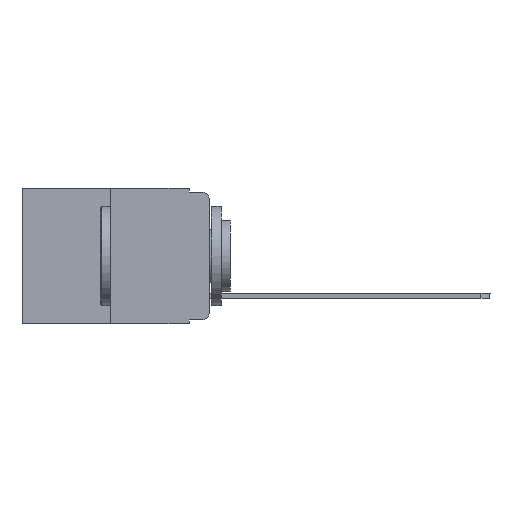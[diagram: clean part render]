
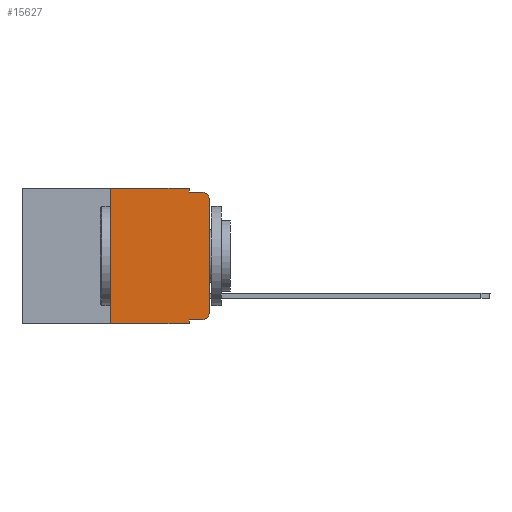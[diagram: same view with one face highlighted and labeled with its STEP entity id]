
A CAD part, left-side view. The second image highlights one B-rep face of the part: STEP entity #15627.
In plain terms, the highlighted planar face has unit normal (-1, 0, 0).
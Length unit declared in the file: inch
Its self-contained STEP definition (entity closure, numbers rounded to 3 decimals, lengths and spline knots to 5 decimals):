
#507 = CARTESIAN_POINT ( 'NONE',  ( 0., 0.051, 0. ) ) ;
#781 = EDGE_CURVE ( 'NONE', #1619, #7245, #6989, .T. ) ;
#1125 = DIRECTION ( 'NONE',  ( 0., 0., 1. ) ) ;
#1319 = VERTEX_POINT ( 'NONE', #2428 ) ;
#1418 = VECTOR ( 'NONE', #8610, 39.37008 ) ;
#1614 = ORIENTED_EDGE ( 'NONE', *, *, #6108, .T. ) ;
#1619 = VERTEX_POINT ( 'NONE', #7873 ) ;
#1660 = VERTEX_POINT ( 'NONE', #12229 ) ;
#1692 = VERTEX_POINT ( 'NONE', #3944 ) ;
#1760 = VECTOR ( 'NONE', #5339, 39.37008 ) ;
#1814 = EDGE_LOOP ( 'NONE', ( #13357, #5194, #2889, #8014, #16266, #16186, #7702, #11370, #1614, #3317 ) ) ;
#1961 = EDGE_CURVE ( 'NONE', #1660, #7245, #17568, .T. ) ;
#2119 = LINE ( 'NONE', #9915, #14086 ) ;
#2248 = EDGE_CURVE ( 'NONE', #11110, #13710, #10597, .T. ) ;
#2272 = CARTESIAN_POINT ( 'NONE',  ( 0., 0.473, -0.343 ) ) ;
#2428 = CARTESIAN_POINT ( 'NONE',  ( 0., 0.25, 0. ) ) ;
#2456 = FACE_OUTER_BOUND ( 'NONE', #1814, .T. ) ;
#2745 = CARTESIAN_POINT ( 'NONE',  ( 0., 0., -0.03 ) ) ;
#2828 = CARTESIAN_POINT ( 'NONE',  ( 0., 0.02, -0.01 ) ) ;
#2889 = ORIENTED_EDGE ( 'NONE', *, *, #11611, .F. ) ;
#3049 = VECTOR ( 'NONE', #4630, 39.37008 ) ;
#3073 = LINE ( 'NONE', #17088, #6129 ) ;
#3238 = LINE ( 'NONE', #5280, #1760 ) ;
#3317 = ORIENTED_EDGE ( 'NONE', *, *, #2248, .T. ) ;
#3724 = PLANE ( 'NONE',  #8675 ) ;
#3820 = AXIS2_PLACEMENT_3D ( 'NONE', #6805, #5267, #3923 ) ;
#3923 = DIRECTION ( 'NONE',  ( 0., 0., -1. ) ) ;
#3944 = CARTESIAN_POINT ( 'NONE',  ( 0., 0.051, -0.01 ) ) ;
#3973 = DIRECTION ( 'NONE',  ( 1., 0., 0. ) ) ;
#4630 = DIRECTION ( 'NONE',  ( 0., 0., -1. ) ) ;
#4683 = DIRECTION ( 'NONE',  ( 0., 0., -1. ) ) ;
#5143 = EDGE_CURVE ( 'NONE', #1319, #16774, #6836, .T. ) ;
#5194 = ORIENTED_EDGE ( 'NONE', *, *, #5973, .T. ) ;
#5267 = DIRECTION ( 'NONE',  ( -1., 0., 0. ) ) ;
#5280 = CARTESIAN_POINT ( 'NONE',  ( 0., 0.051, -0.01 ) ) ;
#5283 = VERTEX_POINT ( 'NONE', #2828 ) ;
#5339 = DIRECTION ( 'NONE',  ( 0., -1., 0. ) ) ;
#5973 = EDGE_CURVE ( 'NONE', #14614, #5283, #11148, .T. ) ;
#6108 = EDGE_CURVE ( 'NONE', #1619, #11110, #13962, .T. ) ;
#6129 = VECTOR ( 'NONE', #4683, 39.37008 ) ;
#6805 = CARTESIAN_POINT ( 'NONE',  ( 0., 0.02, -0.313 ) ) ;
#6836 = LINE ( 'NONE', #11260, #1418 ) ;
#6989 = LINE ( 'NONE', #507, #3049 ) ;
#7245 = VERTEX_POINT ( 'NONE', #16845 ) ;
#7702 = ORIENTED_EDGE ( 'NONE', *, *, #1961, .T. ) ;
#7873 = CARTESIAN_POINT ( 'NONE',  ( 0., 0.051, -0.333 ) ) ;
#7917 = DIRECTION ( 'NONE',  ( 0., -1., 0. ) ) ;
#8014 = ORIENTED_EDGE ( 'NONE', *, *, #16115, .F. ) ;
#8610 = DIRECTION ( 'NONE',  ( 0., -1., 0. ) ) ;
#8675 = AXIS2_PLACEMENT_3D ( 'NONE', #10785, #3973, #16370 ) ;
#9348 = AXIS2_PLACEMENT_3D ( 'NONE', #14844, #10708, #13522 ) ;
#9357 = CARTESIAN_POINT ( 'NONE',  ( 0., 0.25, 0. ) ) ;
#9858 = DIRECTION ( 'NONE',  ( 0., 0., 1. ) ) ;
#9915 = CARTESIAN_POINT ( 'NONE',  ( 0., 0., 0. ) ) ;
#10597 = CIRCLE ( 'NONE', #3820, 0.02 ) ;
#10708 = DIRECTION ( 'NONE',  ( -1., 0., 0. ) ) ;
#10785 = CARTESIAN_POINT ( 'NONE',  ( 0., 0.473, 0. ) ) ;
#11110 = VERTEX_POINT ( 'NONE', #15625 ) ;
#11136 = VECTOR ( 'NONE', #7917, 39.37008 ) ;
#11148 = CIRCLE ( 'NONE', #9348, 0.02 ) ;
#11236 = VECTOR ( 'NONE', #1125, 39.37008 ) ;
#11260 = CARTESIAN_POINT ( 'NONE',  ( 0., 0.473, 0. ) ) ;
#11370 = ORIENTED_EDGE ( 'NONE', *, *, #781, .F. ) ;
#11430 = CARTESIAN_POINT ( 'NONE',  ( 0., 0., -0.313 ) ) ;
#11611 = EDGE_CURVE ( 'NONE', #1692, #5283, #3238, .T. ) ;
#12091 = CARTESIAN_POINT ( 'NONE',  ( 0., 0.051, -0.333 ) ) ;
#12229 = CARTESIAN_POINT ( 'NONE',  ( 0., 0.25, -0.343 ) ) ;
#13121 = CARTESIAN_POINT ( 'NONE',  ( 0., 0.051, 0. ) ) ;
#13357 = ORIENTED_EDGE ( 'NONE', *, *, #13647, .T. ) ;
#13522 = DIRECTION ( 'NONE',  ( 0., 0., -1. ) ) ;
#13647 = EDGE_CURVE ( 'NONE', #13710, #14614, #2119, .T. ) ;
#13710 = VERTEX_POINT ( 'NONE', #11430 ) ;
#13887 = VECTOR ( 'NONE', #14554, 39.37008 ) ;
#13962 = LINE ( 'NONE', #12091, #11136 ) ;
#14050 = EDGE_CURVE ( 'NONE', #1660, #1319, #16880, .T. ) ;
#14086 = VECTOR ( 'NONE', #9858, 39.37008 ) ;
#14554 = DIRECTION ( 'NONE',  ( 0., -1., 0. ) ) ;
#14614 = VERTEX_POINT ( 'NONE', #2745 ) ;
#14844 = CARTESIAN_POINT ( 'NONE',  ( 0., 0.02, -0.03 ) ) ;
#15625 = CARTESIAN_POINT ( 'NONE',  ( 0., 0.02, -0.333 ) ) ;
#15627 = ADVANCED_FACE ( 'NONE', ( #2456 ), #3724, .F. ) ;
#16115 = EDGE_CURVE ( 'NONE', #16774, #1692, #3073, .T. ) ;
#16186 = ORIENTED_EDGE ( 'NONE', *, *, #14050, .F. ) ;
#16266 = ORIENTED_EDGE ( 'NONE', *, *, #5143, .F. ) ;
#16370 = DIRECTION ( 'NONE',  ( 0., 0., -1. ) ) ;
#16774 = VERTEX_POINT ( 'NONE', #13121 ) ;
#16845 = CARTESIAN_POINT ( 'NONE',  ( 0., 0.051, -0.343 ) ) ;
#16880 = LINE ( 'NONE', #9357, #11236 ) ;
#17088 = CARTESIAN_POINT ( 'NONE',  ( 0., 0.051, 0. ) ) ;
#17568 = LINE ( 'NONE', #2272, #13887 ) ;
